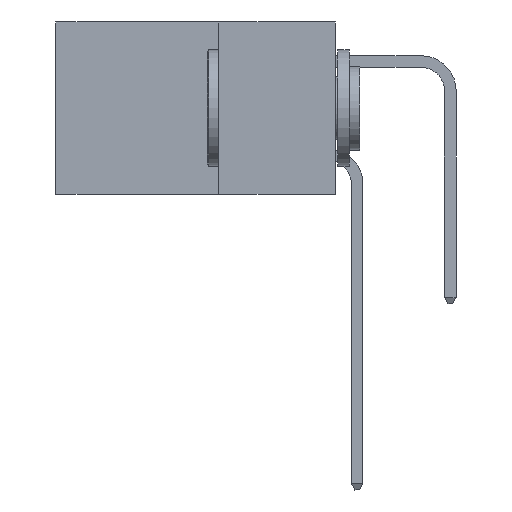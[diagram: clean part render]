
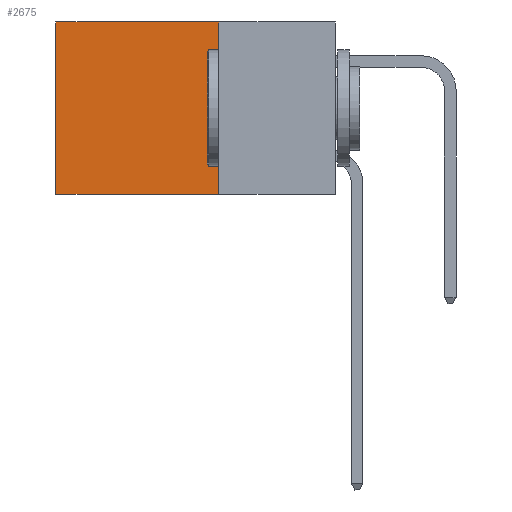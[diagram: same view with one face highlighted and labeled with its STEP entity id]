
A CAD part, left-side view. The second image highlights one B-rep face of the part: STEP entity #2675.
In plain terms, the highlighted planar face has unit normal (-1, 0, 0).
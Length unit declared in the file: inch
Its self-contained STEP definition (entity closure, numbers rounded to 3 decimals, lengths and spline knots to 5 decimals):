
#1376 = PLANE ( 'NONE',  #16418 ) ;
#1899 = ORIENTED_EDGE ( 'NONE', *, *, #13699, .F. ) ;
#2146 = EDGE_CURVE ( 'NONE', #33890, #6904, #21115, .T. ) ;
#2247 = VERTEX_POINT ( 'NONE', #25972 ) ;
#2393 = CARTESIAN_POINT ( 'NONE',  ( 0.2875, 0.6, 0. ) ) ;
#2675 = ADVANCED_FACE ( 'NONE', ( #25221 ), #1376, .F. ) ;
#4112 = DIRECTION ( 'NONE',  ( 0., 1., 0. ) ) ;
#4692 = ORIENTED_EDGE ( 'NONE', *, *, #2146, .T. ) ;
#6904 = VERTEX_POINT ( 'NONE', #29622 ) ;
#7752 = EDGE_CURVE ( 'NONE', #6904, #34501, #8200, .T. ) ;
#8200 = LINE ( 'NONE', #2393, #21558 ) ;
#9307 = CARTESIAN_POINT ( 'NONE',  ( 0.2875, 0.25, 0. ) ) ;
#9840 = CARTESIAN_POINT ( 'NONE',  ( 0.2875, 0.25, 0. ) ) ;
#9955 = DIRECTION ( 'NONE',  ( 0., 0., -1. ) ) ;
#12085 = LINE ( 'NONE', #31086, #23774 ) ;
#12233 = CARTESIAN_POINT ( 'NONE',  ( 0.2875, 0.25, 0. ) ) ;
#13699 = EDGE_CURVE ( 'NONE', #33890, #2247, #25768, .T. ) ;
#15676 = VECTOR ( 'NONE', #22941, 39.37008 ) ;
#16418 = AXIS2_PLACEMENT_3D ( 'NONE', #9840, #17879, #9955 ) ;
#17879 = DIRECTION ( 'NONE',  ( 1., 0., 0. ) ) ;
#18609 = EDGE_CURVE ( 'NONE', #2247, #34501, #12085, .T. ) ;
#21115 = LINE ( 'NONE', #9307, #15676 ) ;
#21558 = VECTOR ( 'NONE', #24915, 39.37008 ) ;
#22030 = VECTOR ( 'NONE', #22955, 39.37008 ) ;
#22606 = CARTESIAN_POINT ( 'NONE',  ( 0.2875, 0.6, -0.37 ) ) ;
#22941 = DIRECTION ( 'NONE',  ( 0., 1., 0. ) ) ;
#22955 = DIRECTION ( 'NONE',  ( 0., 0., -1. ) ) ;
#23774 = VECTOR ( 'NONE', #4112, 39.37008 ) ;
#24647 = EDGE_LOOP ( 'NONE', ( #33140, #34093, #1899, #4692 ) ) ;
#24915 = DIRECTION ( 'NONE',  ( 0., 0., -1. ) ) ;
#25221 = FACE_OUTER_BOUND ( 'NONE', #24647, .T. ) ;
#25768 = LINE ( 'NONE', #12233, #22030 ) ;
#25972 = CARTESIAN_POINT ( 'NONE',  ( 0.2875, 0.25, -0.37 ) ) ;
#29622 = CARTESIAN_POINT ( 'NONE',  ( 0.2875, 0.6, 0. ) ) ;
#31086 = CARTESIAN_POINT ( 'NONE',  ( 0.2875, 0.25, -0.37 ) ) ;
#31401 = CARTESIAN_POINT ( 'NONE',  ( 0.2875, 0.25, 0. ) ) ;
#33140 = ORIENTED_EDGE ( 'NONE', *, *, #7752, .T. ) ;
#33890 = VERTEX_POINT ( 'NONE', #31401 ) ;
#34093 = ORIENTED_EDGE ( 'NONE', *, *, #18609, .F. ) ;
#34501 = VERTEX_POINT ( 'NONE', #22606 ) ;
